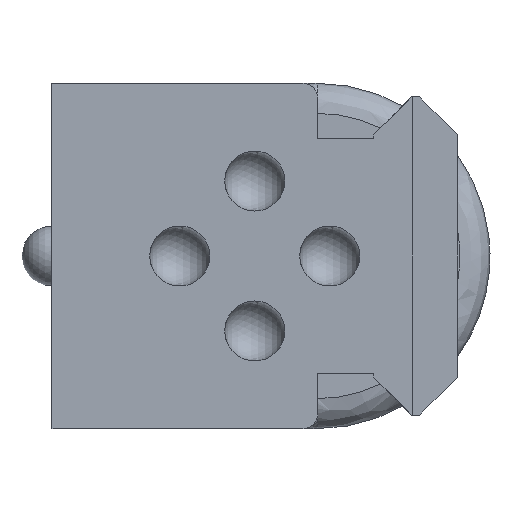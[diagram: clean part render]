
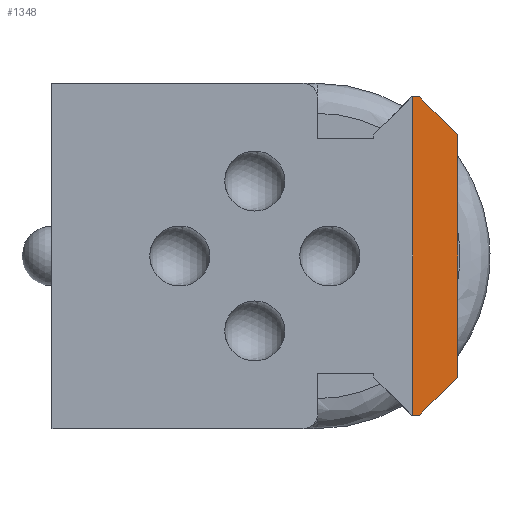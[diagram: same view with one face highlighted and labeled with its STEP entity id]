
A CAD part, front view. The second image highlights one B-rep face of the part: STEP entity #1348.
In plain terms, the highlighted planar face has unit normal (0, -1, 0).
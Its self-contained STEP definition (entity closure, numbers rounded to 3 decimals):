
#26 = EDGE_CURVE ( 'NONE', #2959, #1237, #2423, .T. ) ;
#250 = CARTESIAN_POINT ( 'NONE',  ( -95.68, -90.882, 15.152 ) ) ;
#299 = DIRECTION ( 'NONE',  ( 0., 0., 1. ) ) ;
#320 = DIRECTION ( 'NONE',  ( 0.707, 0., 0.707 ) ) ;
#410 = VECTOR ( 'NONE', #550, 1000. ) ;
#421 = LINE ( 'NONE', #2394, #410 ) ;
#435 = CARTESIAN_POINT ( 'NONE',  ( -98.207, -90.882, 15.152 ) ) ;
#550 = DIRECTION ( 'NONE',  ( 1., 0., 0. ) ) ;
#610 = DIRECTION ( 'NONE',  ( 0., 0., 1. ) ) ;
#709 = EDGE_CURVE ( 'NONE', #2491, #2929, #1591, .T. ) ;
#780 = EDGE_CURVE ( 'NONE', #1014, #1113, #1508, .T. ) ;
#829 = ORIENTED_EDGE ( 'NONE', *, *, #1105, .T. ) ;
#935 = DIRECTION ( 'NONE',  ( 1., 0., 0. ) ) ;
#974 = FACE_OUTER_BOUND ( 'NONE', #1417, .T. ) ;
#1011 = CARTESIAN_POINT ( 'NONE',  ( -97.102, -90.882, -4.952 ) ) ;
#1014 = VERTEX_POINT ( 'NONE', #2126 ) ;
#1088 = LINE ( 'NONE', #2338, #1117 ) ;
#1105 = EDGE_CURVE ( 'NONE', #2929, #2959, #1263, .T. ) ;
#1113 = VERTEX_POINT ( 'NONE', #1973 ) ;
#1117 = VECTOR ( 'NONE', #935, 1000. ) ;
#1156 = CARTESIAN_POINT ( 'NONE',  ( -95.68, -90.882, -3.53 ) ) ;
#1167 = CARTESIAN_POINT ( 'NONE',  ( -95.68, -90.882, 12.625 ) ) ;
#1202 = ORIENTED_EDGE ( 'NONE', *, *, #26, .T. ) ;
#1237 = VERTEX_POINT ( 'NONE', #435 ) ;
#1240 = VECTOR ( 'NONE', #299, 1000. ) ;
#1247 = EDGE_CURVE ( 'NONE', #1014, #2491, #1088, .T. ) ;
#1254 = AXIS2_PLACEMENT_3D ( 'NONE', #2431, #1288, #2833 ) ;
#1263 = LINE ( 'NONE', #250, #1240 ) ;
#1288 = DIRECTION ( 'NONE',  ( 0., 1., 0. ) ) ;
#1348 = ADVANCED_FACE ( 'NONE', ( #974 ), #1990, .F. ) ;
#1417 = EDGE_LOOP ( 'NONE', ( #2831, #829, #1202, #1971, #2738, #2462 ) ) ;
#1508 = LINE ( 'NONE', #2021, #1552 ) ;
#1529 = DIRECTION ( 'NONE',  ( -0.707, 0., 0.707 ) ) ;
#1543 = CARTESIAN_POINT ( 'NONE',  ( -97.102, -90.882, 14.047 ) ) ;
#1552 = VECTOR ( 'NONE', #610, 1000. ) ;
#1579 = VECTOR ( 'NONE', #320, 1000. ) ;
#1591 = LINE ( 'NONE', #1011, #1579 ) ;
#1971 = ORIENTED_EDGE ( 'NONE', *, *, #2101, .F. ) ;
#1973 = CARTESIAN_POINT ( 'NONE',  ( -98.677, -90.882, 15.152 ) ) ;
#1990 = PLANE ( 'NONE',  #1254 ) ;
#2021 = CARTESIAN_POINT ( 'NONE',  ( -98.677, -90.882, 15.152 ) ) ;
#2101 = EDGE_CURVE ( 'NONE', #1113, #1237, #421, .T. ) ;
#2126 = CARTESIAN_POINT ( 'NONE',  ( -98.677, -90.882, -6.057 ) ) ;
#2318 = CARTESIAN_POINT ( 'NONE',  ( -98.207, -90.882, -6.057 ) ) ;
#2338 = CARTESIAN_POINT ( 'NONE',  ( -98.677, -90.882, -6.057 ) ) ;
#2394 = CARTESIAN_POINT ( 'NONE',  ( -98.677, -90.882, 15.152 ) ) ;
#2423 = LINE ( 'NONE', #1543, #2483 ) ;
#2431 = CARTESIAN_POINT ( 'NONE',  ( -98.677, -90.882, 15.152 ) ) ;
#2462 = ORIENTED_EDGE ( 'NONE', *, *, #1247, .T. ) ;
#2483 = VECTOR ( 'NONE', #1529, 1000. ) ;
#2491 = VERTEX_POINT ( 'NONE', #2318 ) ;
#2738 = ORIENTED_EDGE ( 'NONE', *, *, #780, .F. ) ;
#2831 = ORIENTED_EDGE ( 'NONE', *, *, #709, .T. ) ;
#2833 = DIRECTION ( 'NONE',  ( 0., 0., 1. ) ) ;
#2929 = VERTEX_POINT ( 'NONE', #1156 ) ;
#2959 = VERTEX_POINT ( 'NONE', #1167 ) ;
